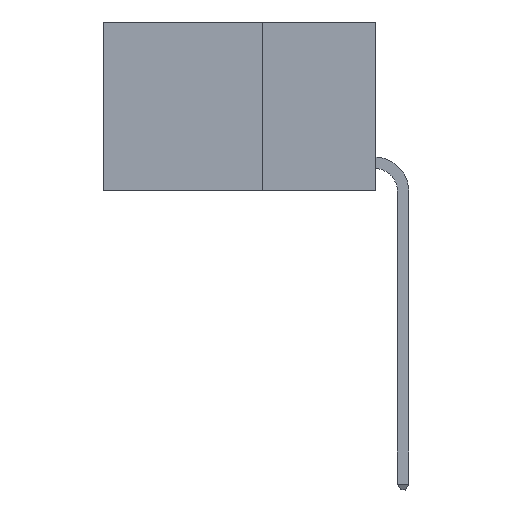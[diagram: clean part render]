
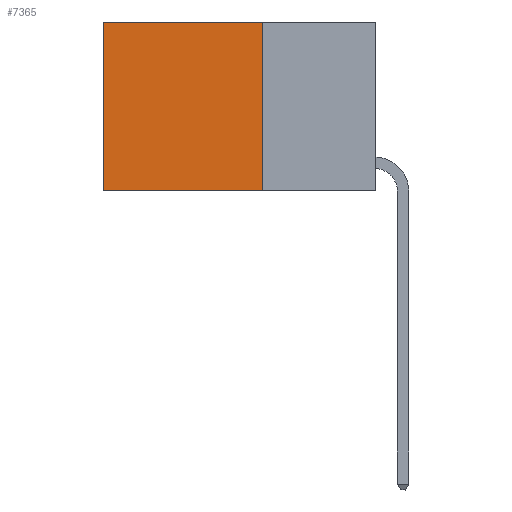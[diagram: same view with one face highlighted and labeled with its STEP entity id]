
A CAD part, left-side view. The second image highlights one B-rep face of the part: STEP entity #7365.
In plain terms, the highlighted planar face has unit normal (-1, 0, 0).
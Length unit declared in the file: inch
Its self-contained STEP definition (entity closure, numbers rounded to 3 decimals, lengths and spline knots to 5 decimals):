
#24 = EDGE_LOOP ( 'NONE', ( #8630, #129, #4023, #5383 ) ) ;
#129 = ORIENTED_EDGE ( 'NONE', *, *, #2946, .F. ) ;
#272 = EDGE_CURVE ( 'NONE', #3295, #2913, #594, .T. ) ;
#334 = PLANE ( 'NONE',  #7517 ) ;
#594 = LINE ( 'NONE', #4336, #873 ) ;
#873 = VECTOR ( 'NONE', #3649, 39.37008 ) ;
#911 = CARTESIAN_POINT ( 'NONE',  ( 0.2625, 0.25, 0. ) ) ;
#1206 = FACE_OUTER_BOUND ( 'NONE', #24, .T. ) ;
#1935 = VERTEX_POINT ( 'NONE', #3228 ) ;
#2913 = VERTEX_POINT ( 'NONE', #5321 ) ;
#2946 = EDGE_CURVE ( 'NONE', #4204, #1935, #6025, .T. ) ;
#2969 = VECTOR ( 'NONE', #5863, 39.37008 ) ;
#3228 = CARTESIAN_POINT ( 'NONE',  ( 0.2625, 0.6, -0.37 ) ) ;
#3295 = VERTEX_POINT ( 'NONE', #6977 ) ;
#3649 = DIRECTION ( 'NONE',  ( 0., 1., 0. ) ) ;
#3993 = CARTESIAN_POINT ( 'NONE',  ( 0.2625, 0.25, 0. ) ) ;
#4023 = ORIENTED_EDGE ( 'NONE', *, *, #8434, .F. ) ;
#4204 = VERTEX_POINT ( 'NONE', #6640 ) ;
#4336 = CARTESIAN_POINT ( 'NONE',  ( 0.2625, 0.25, 0. ) ) ;
#4597 = DIRECTION ( 'NONE',  ( 0., 1., 0. ) ) ;
#4682 = DIRECTION ( 'NONE',  ( 0., 0., -1. ) ) ;
#5015 = CARTESIAN_POINT ( 'NONE',  ( 0.2625, 0.25, -0.37 ) ) ;
#5321 = CARTESIAN_POINT ( 'NONE',  ( 0.2625, 0.6, 0. ) ) ;
#5383 = ORIENTED_EDGE ( 'NONE', *, *, #272, .T. ) ;
#5863 = DIRECTION ( 'NONE',  ( 0., 0., -1. ) ) ;
#6025 = LINE ( 'NONE', #5015, #6662 ) ;
#6298 = LINE ( 'NONE', #6639, #8111 ) ;
#6639 = CARTESIAN_POINT ( 'NONE',  ( 0.2625, 0.6, 0. ) ) ;
#6640 = CARTESIAN_POINT ( 'NONE',  ( 0.2625, 0.25, -0.37 ) ) ;
#6662 = VECTOR ( 'NONE', #4597, 39.37008 ) ;
#6977 = CARTESIAN_POINT ( 'NONE',  ( 0.2625, 0.25, 0. ) ) ;
#7365 = ADVANCED_FACE ( 'NONE', ( #1206 ), #334, .F. ) ;
#7517 = AXIS2_PLACEMENT_3D ( 'NONE', #3993, #8806, #4682 ) ;
#8111 = VECTOR ( 'NONE', #8643, 39.37008 ) ;
#8312 = LINE ( 'NONE', #911, #2969 ) ;
#8434 = EDGE_CURVE ( 'NONE', #3295, #4204, #8312, .T. ) ;
#8452 = EDGE_CURVE ( 'NONE', #2913, #1935, #6298, .T. ) ;
#8630 = ORIENTED_EDGE ( 'NONE', *, *, #8452, .T. ) ;
#8643 = DIRECTION ( 'NONE',  ( 0., 0., -1. ) ) ;
#8806 = DIRECTION ( 'NONE',  ( 1., 0., 0. ) ) ;
